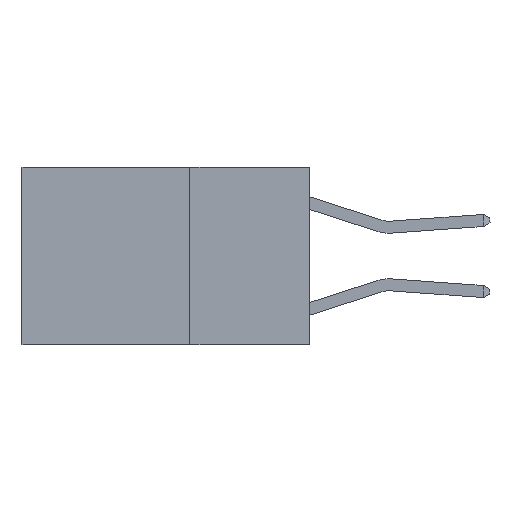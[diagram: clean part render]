
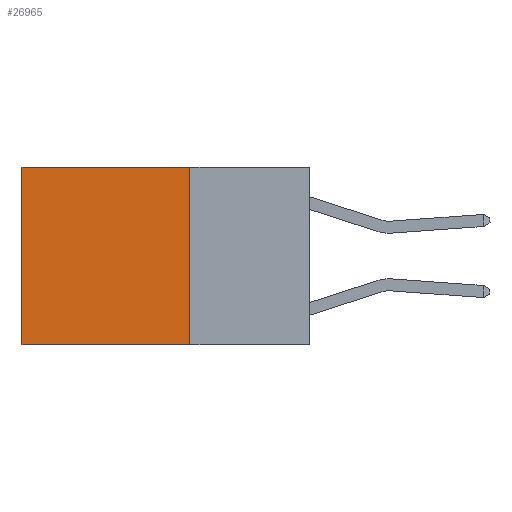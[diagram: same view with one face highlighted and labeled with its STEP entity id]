
A CAD part, left-side view. The second image highlights one B-rep face of the part: STEP entity #26965.
In plain terms, the highlighted planar face has unit normal (-1, 0, 0).
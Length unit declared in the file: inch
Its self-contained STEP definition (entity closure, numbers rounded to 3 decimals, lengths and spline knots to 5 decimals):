
#66 = LINE ( 'NONE', #11811, #28344 ) ;
#433 = DIRECTION ( 'NONE',  ( 0., 1., 0. ) ) ;
#1551 = PLANE ( 'NONE',  #6757 ) ;
#2152 = LINE ( 'NONE', #23453, #25764 ) ;
#3450 = CARTESIAN_POINT ( 'NONE',  ( 0.2625, 0.6, -0.37 ) ) ;
#4156 = VERTEX_POINT ( 'NONE', #10952 ) ;
#4946 = EDGE_CURVE ( 'NONE', #11738, #18627, #66, .T. ) ;
#6130 = DIRECTION ( 'NONE',  ( 1., 0., 0. ) ) ;
#6757 = AXIS2_PLACEMENT_3D ( 'NONE', #17532, #6130, #22143 ) ;
#7409 = ORIENTED_EDGE ( 'NONE', *, *, #27355, .T. ) ;
#8445 = EDGE_LOOP ( 'NONE', ( #7409, #20613, #19295, #14764 ) ) ;
#8601 = VECTOR ( 'NONE', #14466, 39.37008 ) ;
#9319 = LINE ( 'NONE', #18950, #8601 ) ;
#9709 = DIRECTION ( 'NONE',  ( 0., 0., -1. ) ) ;
#10952 = CARTESIAN_POINT ( 'NONE',  ( 0.2625, 0.25, 0. ) ) ;
#11738 = VERTEX_POINT ( 'NONE', #12213 ) ;
#11749 = CARTESIAN_POINT ( 'NONE',  ( 0.2625, 0.25, 0. ) ) ;
#11811 = CARTESIAN_POINT ( 'NONE',  ( 0.2625, 0.25, -0.37 ) ) ;
#12209 = EDGE_CURVE ( 'NONE', #4156, #17896, #20678, .T. ) ;
#12213 = CARTESIAN_POINT ( 'NONE',  ( 0.2625, 0.25, -0.37 ) ) ;
#14068 = DIRECTION ( 'NONE',  ( 0., 1., 0. ) ) ;
#14466 = DIRECTION ( 'NONE',  ( 0., 0., -1. ) ) ;
#14764 = ORIENTED_EDGE ( 'NONE', *, *, #12209, .T. ) ;
#17532 = CARTESIAN_POINT ( 'NONE',  ( 0.2625, 0.25, 0. ) ) ;
#17533 = FACE_OUTER_BOUND ( 'NONE', #8445, .T. ) ;
#17657 = CARTESIAN_POINT ( 'NONE',  ( 0.2625, 0.6, 0. ) ) ;
#17896 = VERTEX_POINT ( 'NONE', #17657 ) ;
#18627 = VERTEX_POINT ( 'NONE', #3450 ) ;
#18950 = CARTESIAN_POINT ( 'NONE',  ( 0.2625, 0.25, 0. ) ) ;
#19295 = ORIENTED_EDGE ( 'NONE', *, *, #23159, .F. ) ;
#19938 = VECTOR ( 'NONE', #14068, 39.37008 ) ;
#20613 = ORIENTED_EDGE ( 'NONE', *, *, #4946, .F. ) ;
#20678 = LINE ( 'NONE', #11749, #19938 ) ;
#22143 = DIRECTION ( 'NONE',  ( 0., 0., -1. ) ) ;
#23159 = EDGE_CURVE ( 'NONE', #4156, #11738, #9319, .T. ) ;
#23453 = CARTESIAN_POINT ( 'NONE',  ( 0.2625, 0.6, 0. ) ) ;
#25764 = VECTOR ( 'NONE', #9709, 39.37008 ) ;
#26965 = ADVANCED_FACE ( 'NONE', ( #17533 ), #1551, .F. ) ;
#27355 = EDGE_CURVE ( 'NONE', #17896, #18627, #2152, .T. ) ;
#28344 = VECTOR ( 'NONE', #433, 39.37008 ) ;
